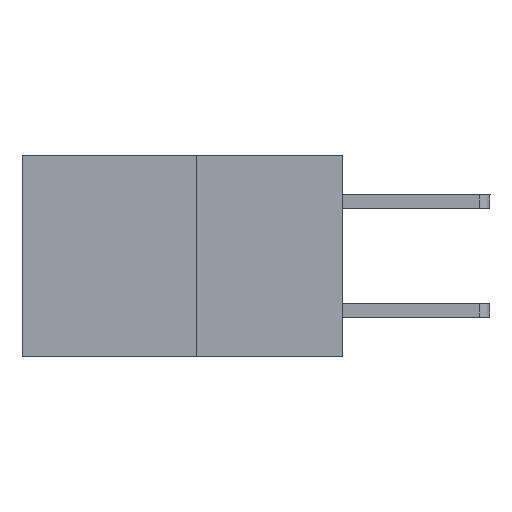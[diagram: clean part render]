
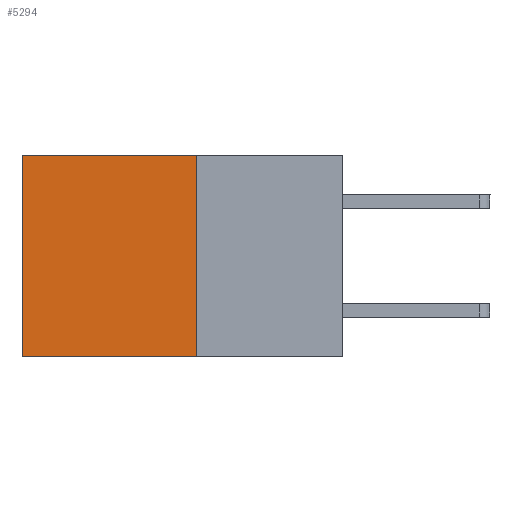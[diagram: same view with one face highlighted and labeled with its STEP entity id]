
A CAD part, left-side view. The second image highlights one B-rep face of the part: STEP entity #5294.
In plain terms, the highlighted planar face has unit normal (-1, 0, 0).
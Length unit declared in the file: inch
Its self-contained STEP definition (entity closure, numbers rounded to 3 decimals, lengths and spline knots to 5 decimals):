
#1452 = AXIS2_PLACEMENT_3D ( 'NONE', #9109, #9074, #3769 ) ;
#1650 = CARTESIAN_POINT ( 'NONE',  ( 0.277, 0.59, 0. ) ) ;
#2318 = ORIENTED_EDGE ( 'NONE', *, *, #8256, .T. ) ;
#2413 = ORIENTED_EDGE ( 'NONE', *, *, #10020, .T. ) ;
#2662 = ORIENTED_EDGE ( 'NONE', *, *, #9945, .F. ) ;
#2951 = CARTESIAN_POINT ( 'NONE',  ( 0.277, 0.59, -0.37 ) ) ;
#3258 = CARTESIAN_POINT ( 'NONE',  ( 0.277, 0.27, 0. ) ) ;
#3406 = CARTESIAN_POINT ( 'NONE',  ( 0.277, 0.27, 0. ) ) ;
#3769 = DIRECTION ( 'NONE',  ( 0., 0., -1. ) ) ;
#4146 = DIRECTION ( 'NONE',  ( 0., 1., 0. ) ) ;
#4209 = CARTESIAN_POINT ( 'NONE',  ( 0.277, 0.27, -0.37 ) ) ;
#4220 = DIRECTION ( 'NONE',  ( 0., 1., 0. ) ) ;
#4599 = DIRECTION ( 'NONE',  ( 0., 0., -1. ) ) ;
#4920 = CARTESIAN_POINT ( 'NONE',  ( 0.277, 0.59, -0.37 ) ) ;
#4955 = LINE ( 'NONE', #7064, #7364 ) ;
#5197 = DIRECTION ( 'NONE',  ( 0., 0., -1. ) ) ;
#5294 = ADVANCED_FACE ( 'NONE', ( #8162 ), #9087, .F. ) ;
#5674 = VECTOR ( 'NONE', #4220, 39.37008 ) ;
#5885 = VERTEX_POINT ( 'NONE', #1650 ) ;
#5989 = VECTOR ( 'NONE', #4146, 39.37008 ) ;
#6484 = EDGE_LOOP ( 'NONE', ( #2318, #2662, #6676, #2413 ) ) ;
#6676 = ORIENTED_EDGE ( 'NONE', *, *, #9044, .F. ) ;
#7064 = CARTESIAN_POINT ( 'NONE',  ( 0.277, 0.27, -0.37 ) ) ;
#7364 = VECTOR ( 'NONE', #5197, 39.37008 ) ;
#7588 = VERTEX_POINT ( 'NONE', #3258 ) ;
#7706 = LINE ( 'NONE', #3406, #5674 ) ;
#7755 = VERTEX_POINT ( 'NONE', #4209 ) ;
#7849 = VECTOR ( 'NONE', #4599, 39.37008 ) ;
#8162 = FACE_OUTER_BOUND ( 'NONE', #6484, .T. ) ;
#8256 = EDGE_CURVE ( 'NONE', #5885, #8678, #9779, .T. ) ;
#8396 = CARTESIAN_POINT ( 'NONE',  ( 0.277, 0.27, -0.37 ) ) ;
#8678 = VERTEX_POINT ( 'NONE', #4920 ) ;
#9044 = EDGE_CURVE ( 'NONE', #7588, #7755, #4955, .T. ) ;
#9074 = DIRECTION ( 'NONE',  ( 1., 0., 0. ) ) ;
#9087 = PLANE ( 'NONE',  #1452 ) ;
#9109 = CARTESIAN_POINT ( 'NONE',  ( 0.277, 0.27, -0.37 ) ) ;
#9779 = LINE ( 'NONE', #2951, #7849 ) ;
#9945 = EDGE_CURVE ( 'NONE', #7755, #8678, #10289, .T. ) ;
#10020 = EDGE_CURVE ( 'NONE', #7588, #5885, #7706, .T. ) ;
#10289 = LINE ( 'NONE', #8396, #5989 ) ;
